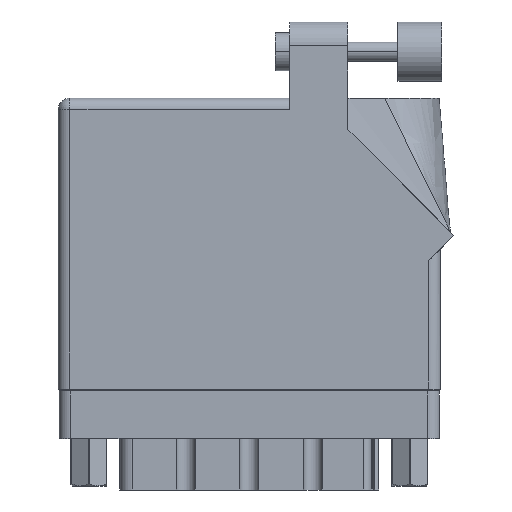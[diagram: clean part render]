
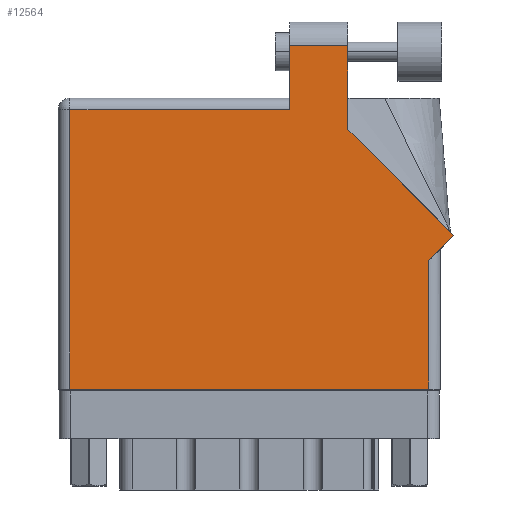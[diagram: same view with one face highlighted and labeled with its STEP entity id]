
A CAD part, front view. The second image highlights one B-rep face of the part: STEP entity #12564.
In plain terms, the highlighted face is planar.
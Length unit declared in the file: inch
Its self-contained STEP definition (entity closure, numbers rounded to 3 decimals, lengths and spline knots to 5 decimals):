
#235 = DIRECTION ( 'NONE',  ( 0., -1., 0. ) ) ;
#653 = VERTEX_POINT ( 'NONE', #12369 ) ;
#973 = DIRECTION ( 'NONE',  ( -1., 0., 0. ) ) ;
#1053 = EDGE_CURVE ( 'NONE', #29158, #42607, #4113, .T. ) ;
#1442 = CARTESIAN_POINT ( 'NONE',  ( 1.948, 0., 0. ) ) ;
#1692 = VECTOR ( 'NONE', #11708, 39.37008 ) ;
#2997 = VERTEX_POINT ( 'NONE', #13021 ) ;
#3003 = VERTEX_POINT ( 'NONE', #41786 ) ;
#3070 = AXIS2_PLACEMENT_3D ( 'NONE', #7151, #14113, #10263 ) ;
#4113 = LINE ( 'NONE', #44364, #20756 ) ;
#4137 = LINE ( 'NONE', #14778, #31374 ) ;
#4717 = DIRECTION ( 'NONE',  ( 0., -1., 0. ) ) ;
#5472 = DIRECTION ( 'NONE',  ( 1., 0., 0. ) ) ;
#6376 = VECTOR ( 'NONE', #973, 39.37008 ) ;
#7151 = CARTESIAN_POINT ( 'NONE',  ( 0., 1.53, 0. ) ) ;
#7204 = ORIENTED_EDGE ( 'NONE', *, *, #20419, .T. ) ;
#8729 = ORIENTED_EDGE ( 'NONE', *, *, #37310, .T. ) ;
#8753 = CARTESIAN_POINT ( 'NONE',  ( 1.217, 1.805, 0. ) ) ;
#9761 = LINE ( 'NONE', #26734, #34172 ) ;
#10157 = ORIENTED_EDGE ( 'NONE', *, *, #40198, .T. ) ;
#10263 = DIRECTION ( 'NONE',  ( -1., 0., 0. ) ) ;
#10312 = CARTESIAN_POINT ( 'NONE',  ( 1.217, 1.805, 0. ) ) ;
#11708 = DIRECTION ( 'NONE',  ( 0., 1., 0. ) ) ;
#12192 = EDGE_CURVE ( 'NONE', #2997, #653, #27772, .T. ) ;
#12369 = CARTESIAN_POINT ( 'NONE',  ( 0.062, 0., 0. ) ) ;
#12506 = DIRECTION ( 'NONE',  ( -1., 0., 0. ) ) ;
#12564 = ADVANCED_FACE ( 'NONE', ( #15451 ), #31982, .F. ) ;
#12735 = ORIENTED_EDGE ( 'NONE', *, *, #30004, .T. ) ;
#13021 = CARTESIAN_POINT ( 'NONE',  ( 0.062, 1.468, 0. ) ) ;
#13983 = CARTESIAN_POINT ( 'NONE',  ( 1.948, 0.675, 0. ) ) ;
#14113 = DIRECTION ( 'NONE',  ( 0., 0., -1. ) ) ;
#14778 = CARTESIAN_POINT ( 'NONE',  ( 1.217, 1.53, 0. ) ) ;
#14795 = EDGE_CURVE ( 'NONE', #32009, #37177, #4137, .T. ) ;
#15009 = VECTOR ( 'NONE', #12506, 39.37008 ) ;
#15223 = CARTESIAN_POINT ( 'NONE',  ( 0.062, 0., 0. ) ) ;
#15413 = DIRECTION ( 'NONE',  ( 0.707, 0.707, 0. ) ) ;
#15451 = FACE_OUTER_BOUND ( 'NONE', #18133, .T. ) ;
#17744 = CARTESIAN_POINT ( 'NONE',  ( 1.524, 1.36442, 0. ) ) ;
#18133 = EDGE_LOOP ( 'NONE', ( #45315, #12735, #26353, #8729, #29220, #10157, #7204, #39942, #44020 ) ) ;
#18374 = EDGE_CURVE ( 'NONE', #42607, #3003, #20794, .T. ) ;
#18542 = CARTESIAN_POINT ( 'NONE',  ( 1.948, 0.737, 0. ) ) ;
#20419 = EDGE_CURVE ( 'NONE', #32015, #29158, #32781, .T. ) ;
#20756 = VECTOR ( 'NONE', #15413, 39.37008 ) ;
#20794 = LINE ( 'NONE', #28582, #28591 ) ;
#22284 = CARTESIAN_POINT ( 'NONE',  ( 1.217, 1.468, 0. ) ) ;
#25037 = LINE ( 'NONE', #41258, #15009 ) ;
#26149 = VECTOR ( 'NONE', #42795, 39.37008 ) ;
#26353 = ORIENTED_EDGE ( 'NONE', *, *, #14795, .T. ) ;
#26621 = EDGE_CURVE ( 'NONE', #3003, #41895, #42852, .T. ) ;
#26734 = CARTESIAN_POINT ( 'NONE',  ( 0., 0., 0. ) ) ;
#27772 = LINE ( 'NONE', #15223, #45003 ) ;
#28582 = CARTESIAN_POINT ( 'NONE',  ( 2.08071, 0.80771, 0. ) ) ;
#28591 = VECTOR ( 'NONE', #31650, 39.37008 ) ;
#29158 = VERTEX_POINT ( 'NONE', #13983 ) ;
#29220 = ORIENTED_EDGE ( 'NONE', *, *, #12192, .T. ) ;
#30004 = EDGE_CURVE ( 'NONE', #41895, #32009, #44183, .T. ) ;
#30081 = CARTESIAN_POINT ( 'NONE',  ( 2.08071, 0.80771, 0. ) ) ;
#31374 = VECTOR ( 'NONE', #235, 39.37008 ) ;
#31650 = DIRECTION ( 'NONE',  ( -0.707, 0.707, 0. ) ) ;
#31982 = PLANE ( 'NONE',  #3070 ) ;
#32009 = VERTEX_POINT ( 'NONE', #8753 ) ;
#32015 = VERTEX_POINT ( 'NONE', #1442 ) ;
#32781 = LINE ( 'NONE', #18542, #1692 ) ;
#34172 = VECTOR ( 'NONE', #5472, 39.37008 ) ;
#37177 = VERTEX_POINT ( 'NONE', #22284 ) ;
#37310 = EDGE_CURVE ( 'NONE', #37177, #2997, #25037, .T. ) ;
#39942 = ORIENTED_EDGE ( 'NONE', *, *, #1053, .T. ) ;
#40198 = EDGE_CURVE ( 'NONE', #653, #32015, #9761, .T. ) ;
#41258 = CARTESIAN_POINT ( 'NONE',  ( 0., 1.468, 0. ) ) ;
#41786 = CARTESIAN_POINT ( 'NONE',  ( 1.524, 1.36442, 0. ) ) ;
#41895 = VERTEX_POINT ( 'NONE', #43504 ) ;
#42607 = VERTEX_POINT ( 'NONE', #30081 ) ;
#42795 = DIRECTION ( 'NONE',  ( 0., 1., 0. ) ) ;
#42852 = LINE ( 'NONE', #17744, #26149 ) ;
#43504 = CARTESIAN_POINT ( 'NONE',  ( 1.524, 1.805, 0. ) ) ;
#44020 = ORIENTED_EDGE ( 'NONE', *, *, #18374, .T. ) ;
#44183 = LINE ( 'NONE', #10312, #6376 ) ;
#44364 = CARTESIAN_POINT ( 'NONE',  ( 2.01, 0.737, 0. ) ) ;
#45003 = VECTOR ( 'NONE', #4717, 39.37008 ) ;
#45315 = ORIENTED_EDGE ( 'NONE', *, *, #26621, .T. ) ;
